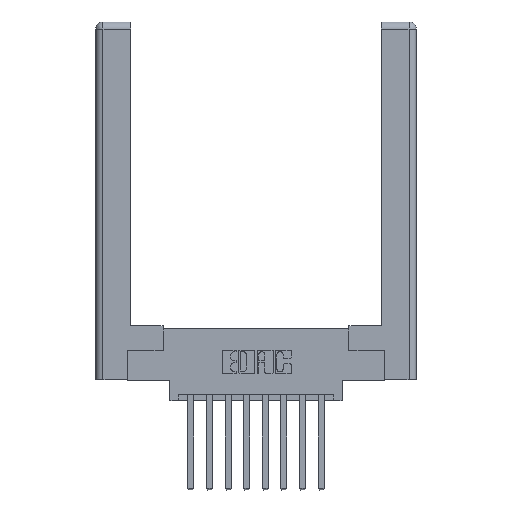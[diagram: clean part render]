
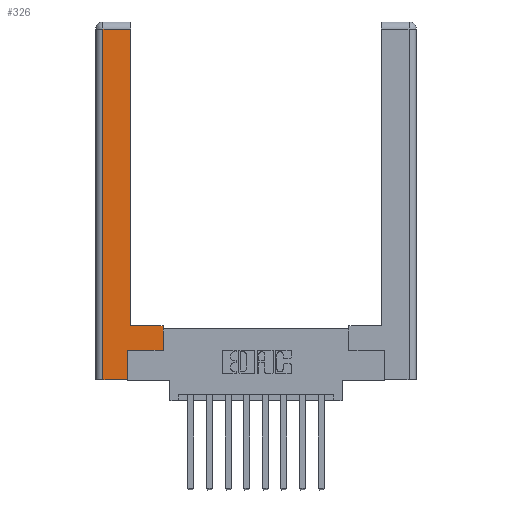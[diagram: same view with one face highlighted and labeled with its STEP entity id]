
A CAD part, top view. The second image highlights one B-rep face of the part: STEP entity #326.
In plain terms, the highlighted planar face has unit normal (0, 0, 1).
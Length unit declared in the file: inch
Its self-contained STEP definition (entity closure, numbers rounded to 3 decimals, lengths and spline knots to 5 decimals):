
#57 = CARTESIAN_POINT ( 'NONE',  ( 0.265, 0., 0. ) ) ;
#124 = VERTEX_POINT ( 'NONE', #4335 ) ;
#311 = EDGE_CURVE ( 'NONE', #8293, #124, #1839, .T. ) ;
#326 = ADVANCED_FACE ( 'NONE', ( #4883 ), #12580, .F. ) ;
#482 = LINE ( 'NONE', #57, #1446 ) ;
#490 = VERTEX_POINT ( 'NONE', #4155 ) ;
#935 = CARTESIAN_POINT ( 'NONE',  ( 0.0615, 2.94, 0. ) ) ;
#937 = VECTOR ( 'NONE', #11464, 39.37008 ) ;
#948 = ORIENTED_EDGE ( 'NONE', *, *, #11716, .T. ) ;
#1037 = VERTEX_POINT ( 'NONE', #12177 ) ;
#1250 = ORIENTED_EDGE ( 'NONE', *, *, #3858, .T. ) ;
#1446 = VECTOR ( 'NONE', #10126, 39.37008 ) ;
#1578 = DIRECTION ( 'NONE',  ( 0., 0., -1. ) ) ;
#1839 = LINE ( 'NONE', #3386, #5041 ) ;
#1953 = VECTOR ( 'NONE', #7826, 39.37008 ) ;
#2023 = AXIS2_PLACEMENT_3D ( 'NONE', #10588, #1578, #10753 ) ;
#2108 = ORIENTED_EDGE ( 'NONE', *, *, #7269, .T. ) ;
#3171 = LINE ( 'NONE', #11580, #11447 ) ;
#3386 = CARTESIAN_POINT ( 'NONE',  ( 0.295, 3., 0. ) ) ;
#3674 = LINE ( 'NONE', #7302, #7973 ) ;
#3676 = LINE ( 'NONE', #6330, #937 ) ;
#3808 = CARTESIAN_POINT ( 'NONE',  ( 0.295, 0.45, 0. ) ) ;
#3858 = EDGE_CURVE ( 'NONE', #8119, #1037, #3674, .T. ) ;
#3943 = CARTESIAN_POINT ( 'NONE',  ( 0.0615, 0., 0. ) ) ;
#4129 = DIRECTION ( 'NONE',  ( 0., 1., 0. ) ) ;
#4155 = CARTESIAN_POINT ( 'NONE',  ( 0.265, 0., 0. ) ) ;
#4335 = CARTESIAN_POINT ( 'NONE',  ( 0.295, 2.94, 0. ) ) ;
#4883 = FACE_OUTER_BOUND ( 'NONE', #12808, .T. ) ;
#4884 = ORIENTED_EDGE ( 'NONE', *, *, #7082, .T. ) ;
#5041 = VECTOR ( 'NONE', #5463, 39.37008 ) ;
#5117 = CARTESIAN_POINT ( 'NONE',  ( 0.265, 0.245, 0. ) ) ;
#5463 = DIRECTION ( 'NONE',  ( 0., 1., 0. ) ) ;
#5548 = EDGE_CURVE ( 'NONE', #5944, #8119, #3171, .T. ) ;
#5786 = CARTESIAN_POINT ( 'NONE',  ( 0.565, 0.245, 0. ) ) ;
#5817 = LINE ( 'NONE', #935, #9119 ) ;
#5944 = VERTEX_POINT ( 'NONE', #5117 ) ;
#6151 = CARTESIAN_POINT ( 'NONE',  ( 0.295, 0.45, 0. ) ) ;
#6330 = CARTESIAN_POINT ( 'NONE',  ( 0.0615, 0., 0. ) ) ;
#6530 = DIRECTION ( 'NONE',  ( 1., 0., 0. ) ) ;
#7082 = EDGE_CURVE ( 'NONE', #8793, #490, #482, .T. ) ;
#7172 = ORIENTED_EDGE ( 'NONE', *, *, #5548, .T. ) ;
#7269 = EDGE_CURVE ( 'NONE', #7575, #8793, #3676, .T. ) ;
#7302 = CARTESIAN_POINT ( 'NONE',  ( 0.565, 0.45, 0. ) ) ;
#7575 = VERTEX_POINT ( 'NONE', #10642 ) ;
#7826 = DIRECTION ( 'NONE',  ( -1., 0., 0. ) ) ;
#7973 = VECTOR ( 'NONE', #4129, 39.37008 ) ;
#8119 = VERTEX_POINT ( 'NONE', #5786 ) ;
#8293 = VERTEX_POINT ( 'NONE', #6151 ) ;
#8676 = ORIENTED_EDGE ( 'NONE', *, *, #311, .T. ) ;
#8793 = VERTEX_POINT ( 'NONE', #3943 ) ;
#9119 = VECTOR ( 'NONE', #11057, 39.37008 ) ;
#9587 = ORIENTED_EDGE ( 'NONE', *, *, #10340, .T. ) ;
#10126 = DIRECTION ( 'NONE',  ( 1., 0., 0. ) ) ;
#10340 = EDGE_CURVE ( 'NONE', #490, #5944, #11241, .T. ) ;
#10588 = CARTESIAN_POINT ( 'NONE',  ( 0., 0., 0. ) ) ;
#10642 = CARTESIAN_POINT ( 'NONE',  ( 0.0615, 2.94, 0. ) ) ;
#10753 = DIRECTION ( 'NONE',  ( -1., 0., 0. ) ) ;
#10760 = VECTOR ( 'NONE', #12577, 39.37008 ) ;
#10994 = ORIENTED_EDGE ( 'NONE', *, *, #11735, .T. ) ;
#11057 = DIRECTION ( 'NONE',  ( -1., 0., 0. ) ) ;
#11241 = LINE ( 'NONE', #11654, #10760 ) ;
#11447 = VECTOR ( 'NONE', #6530, 39.37008 ) ;
#11464 = DIRECTION ( 'NONE',  ( 0., -1., 0. ) ) ;
#11580 = CARTESIAN_POINT ( 'NONE',  ( 0.565, 0.245, 0. ) ) ;
#11654 = CARTESIAN_POINT ( 'NONE',  ( 0.265, 0.245, 0. ) ) ;
#11716 = EDGE_CURVE ( 'NONE', #1037, #8293, #12482, .T. ) ;
#11735 = EDGE_CURVE ( 'NONE', #124, #7575, #5817, .T. ) ;
#12177 = CARTESIAN_POINT ( 'NONE',  ( 0.565, 0.45, 0. ) ) ;
#12482 = LINE ( 'NONE', #3808, #1953 ) ;
#12577 = DIRECTION ( 'NONE',  ( 0., 1., 0. ) ) ;
#12580 = PLANE ( 'NONE',  #2023 ) ;
#12808 = EDGE_LOOP ( 'NONE', ( #8676, #10994, #2108, #4884, #9587, #7172, #1250, #948 ) ) ;
